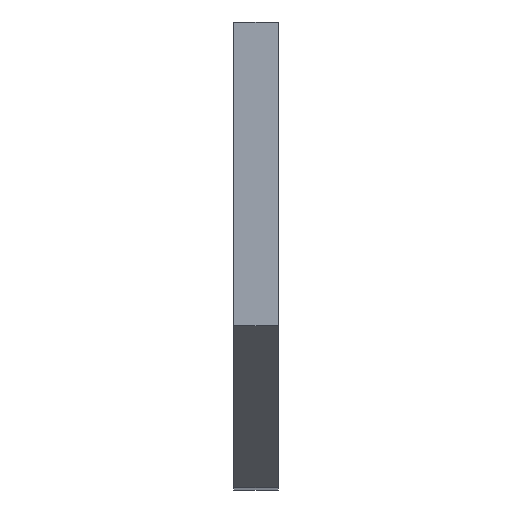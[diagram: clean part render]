
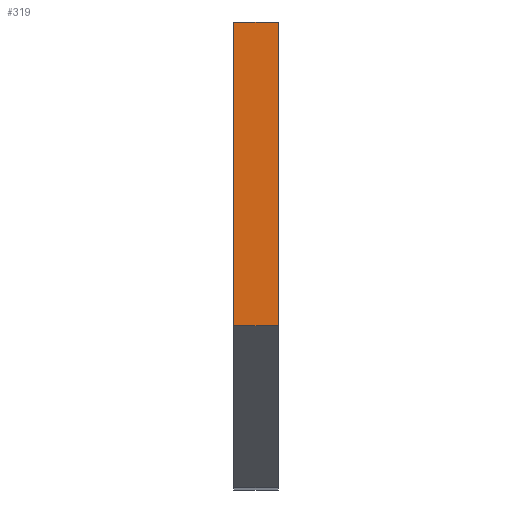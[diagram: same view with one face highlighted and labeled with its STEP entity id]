
A CAD part, top view. The second image highlights one B-rep face of the part: STEP entity #319.
In plain terms, the highlighted planar face has unit normal (0, 0, 1).
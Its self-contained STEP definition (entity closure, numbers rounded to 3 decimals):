
#23 = EDGE_CURVE ( 'NONE', #353, #90, #566, .T. ) ;
#33 = EDGE_CURVE ( 'NONE', #39, #353, #525, .T. ) ;
#39 = VERTEX_POINT ( 'NONE', #344 ) ;
#51 = ORIENTED_EDGE ( 'NONE', *, *, #23, .F. ) ;
#75 = ORIENTED_EDGE ( 'NONE', *, *, #632, .T. ) ;
#90 = VERTEX_POINT ( 'NONE', #303 ) ;
#156 = CARTESIAN_POINT ( 'NONE',  ( 0., 0., 0. ) ) ;
#194 = DIRECTION ( 'NONE',  ( 0., -1., 0. ) ) ;
#236 = CARTESIAN_POINT ( 'NONE',  ( 0., 33.426, 0. ) ) ;
#265 = FACE_OUTER_BOUND ( 'NONE', #571, .T. ) ;
#303 = CARTESIAN_POINT ( 'NONE',  ( 0., 11.608, 0. ) ) ;
#319 = ADVANCED_FACE ( 'NONE', ( #265 ), #460, .F. ) ;
#338 = LINE ( 'NONE', #156, #360 ) ;
#344 = CARTESIAN_POINT ( 'NONE',  ( 3.175, 33.426, 0. ) ) ;
#353 = VERTEX_POINT ( 'NONE', #426 ) ;
#360 = VECTOR ( 'NONE', #194, 1000. ) ;
#390 = DIRECTION ( 'NONE',  ( 0., -1., 0. ) ) ;
#399 = CARTESIAN_POINT ( 'NONE',  ( 3.175, 11.608, 0. ) ) ;
#421 = CARTESIAN_POINT ( 'NONE',  ( 3.175, 0., 0. ) ) ;
#426 = CARTESIAN_POINT ( 'NONE',  ( 3.175, 11.608, 0. ) ) ;
#432 = DIRECTION ( 'NONE',  ( -1., 0., 0. ) ) ;
#454 = DIRECTION ( 'NONE',  ( 0., 1., 0. ) ) ;
#456 = DIRECTION ( 'NONE',  ( 0., 0., -1. ) ) ;
#460 = PLANE ( 'NONE',  #690 ) ;
#463 = CARTESIAN_POINT ( 'NONE',  ( 3.175, 0., 0. ) ) ;
#467 = VECTOR ( 'NONE', #390, 1000. ) ;
#523 = VECTOR ( 'NONE', #432, 1000. ) ;
#525 = LINE ( 'NONE', #421, #467 ) ;
#536 = VERTEX_POINT ( 'NONE', #236 ) ;
#545 = EDGE_CURVE ( 'NONE', #536, #90, #338, .T. ) ;
#566 = LINE ( 'NONE', #399, #523 ) ;
#571 = EDGE_LOOP ( 'NONE', ( #757, #51, #584, #75 ) ) ;
#584 = ORIENTED_EDGE ( 'NONE', *, *, #33, .F. ) ;
#632 = EDGE_CURVE ( 'NONE', #39, #536, #695, .T. ) ;
#634 = DIRECTION ( 'NONE',  ( -1., 0., 0. ) ) ;
#647 = CARTESIAN_POINT ( 'NONE',  ( 3.175, 33.426, 0. ) ) ;
#680 = VECTOR ( 'NONE', #634, 1000. ) ;
#690 = AXIS2_PLACEMENT_3D ( 'NONE', #463, #456, #454 ) ;
#695 = LINE ( 'NONE', #647, #680 ) ;
#757 = ORIENTED_EDGE ( 'NONE', *, *, #545, .T. ) ;
